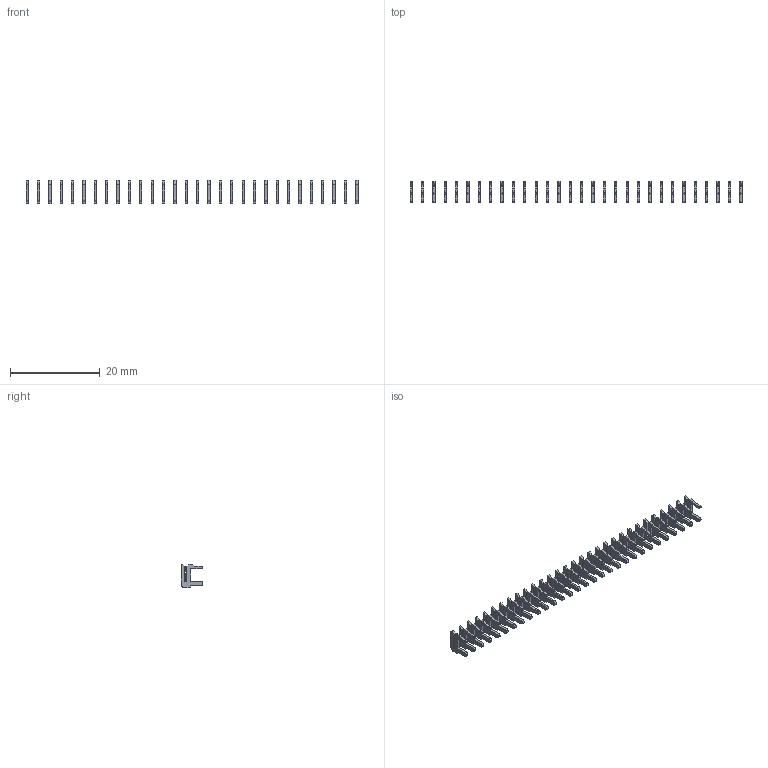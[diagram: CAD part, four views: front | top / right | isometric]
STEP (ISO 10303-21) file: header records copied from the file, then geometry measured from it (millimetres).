
FILE_DESCRIPTION (( 'STEP AP203' ), '1' );
FILE_NAME ('105-030-208-100.STEP', '2020-04-07T23:27:29', ( '' ), ( '' ), 'SwSTEP 2.0', 'SolidWorks 2016', '' );
FILE_SCHEMA (( 'CONFIG_CONTROL_DESIGN' ));
Length unit declared in the file: inch
Products named in the file (2): 105-030-208-100; 100-290-001_100-290-208
Assembly tree (30 placements, depth 2):
  105-030-208-100
    100-290-001_100-290-208  x30
Bounding box: 74.17 x 4.83 x 5.17 mm (x, y, z)
Volume: 206.4 mm3; surface area: 1274.9 mm2
Topology: 30 solids, 30 shells, 750 faces, 2070 edges, 1380 vertices
Faces by surface type: plane 660, cylinder 90
Entity records: 1917 total; most frequent: DIRECTION 191, CARTESIAN_POINT 173, ORIENTED_EDGE 138, LOCAL_TIME 70, DATE_AND_TIME 70, CALENDAR_DATE 70, COORDINATED_UNIVERSAL_TIME_OFFSET 70, EDGE_CURVE 69
